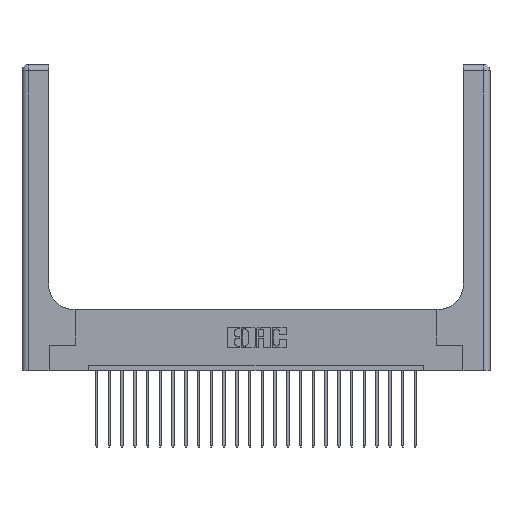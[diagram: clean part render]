
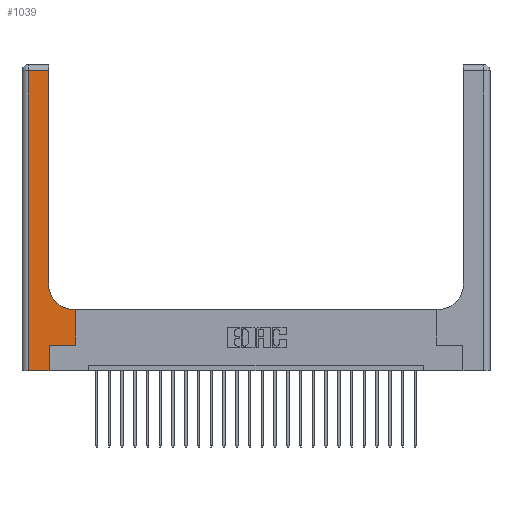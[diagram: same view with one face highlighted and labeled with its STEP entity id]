
A CAD part, top view. The second image highlights one B-rep face of the part: STEP entity #1039.
In plain terms, the highlighted planar face has unit normal (0, 0, 1).
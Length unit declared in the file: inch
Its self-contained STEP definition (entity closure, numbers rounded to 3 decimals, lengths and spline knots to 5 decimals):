
#389 = VERTEX_POINT ( 'NONE', #12969 ) ;
#565 = DIRECTION ( 'NONE',  ( 1., 0., 0. ) ) ;
#596 = EDGE_CURVE ( 'NONE', #2358, #16063, #3542, .T. ) ;
#1039 = ADVANCED_FACE ( 'NONE', ( #17517 ), #15504, .F. ) ;
#1702 = AXIS2_PLACEMENT_3D ( 'NONE', #22422, #6206, #7999 ) ;
#2172 = VECTOR ( 'NONE', #17030, 39.37008 ) ;
#2254 = EDGE_CURVE ( 'NONE', #389, #21819, #23244, .T. ) ;
#2358 = VERTEX_POINT ( 'NONE', #20498 ) ;
#2521 = DIRECTION ( 'NONE',  ( 0., 1., 0. ) ) ;
#2607 = CARTESIAN_POINT ( 'NONE',  ( 0., 0., 0.37 ) ) ;
#3182 = DIRECTION ( 'NONE',  ( 0., 1., 0. ) ) ;
#3448 = EDGE_CURVE ( 'NONE', #3880, #2358, #19218, .T. ) ;
#3542 = LINE ( 'NONE', #15411, #4671 ) ;
#3593 = ORIENTED_EDGE ( 'NONE', *, *, #3448, .T. ) ;
#3880 = VERTEX_POINT ( 'NONE', #18646 ) ;
#4174 = VERTEX_POINT ( 'NONE', #15863 ) ;
#4275 = CARTESIAN_POINT ( 'NONE',  ( 0.265, 0.25, 0.37 ) ) ;
#4594 = CARTESIAN_POINT ( 'NONE',  ( 0., 3., 0.37 ) ) ;
#4671 = VECTOR ( 'NONE', #2521, 39.37008 ) ;
#5484 = VECTOR ( 'NONE', #18751, 39.37008 ) ;
#5961 = VECTOR ( 'NONE', #6491, 39.37008 ) ;
#5964 = EDGE_CURVE ( 'NONE', #13296, #11748, #10240, .T. ) ;
#5990 = ORIENTED_EDGE ( 'NONE', *, *, #5964, .T. ) ;
#6074 = EDGE_CURVE ( 'NONE', #4174, #13296, #15674, .T. ) ;
#6206 = DIRECTION ( 'NONE',  ( 0., 0., -1. ) ) ;
#6491 = DIRECTION ( 'NONE',  ( 0., -1., 0. ) ) ;
#7997 = DIRECTION ( 'NONE',  ( -1., 0., 0. ) ) ;
#7999 = DIRECTION ( 'NONE',  ( 1., 0., 0. ) ) ;
#8484 = ORIENTED_EDGE ( 'NONE', *, *, #16014, .T. ) ;
#8502 = ORIENTED_EDGE ( 'NONE', *, *, #10331, .T. ) ;
#8885 = LINE ( 'NONE', #20473, #5484 ) ;
#8945 = LINE ( 'NONE', #4275, #13223 ) ;
#10072 = DIRECTION ( 'NONE',  ( -1., 0., 0. ) ) ;
#10240 = LINE ( 'NONE', #15080, #22770 ) ;
#10331 = EDGE_CURVE ( 'NONE', #11748, #18157, #20319, .T. ) ;
#11748 = VERTEX_POINT ( 'NONE', #16705 ) ;
#12388 = CARTESIAN_POINT ( 'NONE',  ( 0.26, 0.85, 0.37 ) ) ;
#12969 = CARTESIAN_POINT ( 'NONE',  ( 0.26, 2.94, 0.37 ) ) ;
#13201 = CARTESIAN_POINT ( 'NONE',  ( 0.528, 0.6, 0.37 ) ) ;
#13223 = VECTOR ( 'NONE', #565, 39.37008 ) ;
#13296 = VERTEX_POINT ( 'NONE', #13201 ) ;
#14224 = EDGE_CURVE ( 'NONE', #16063, #4174, #8945, .T. ) ;
#14757 = VECTOR ( 'NONE', #7997, 39.37008 ) ;
#14937 = ORIENTED_EDGE ( 'NONE', *, *, #596, .T. ) ;
#15080 = CARTESIAN_POINT ( 'NONE',  ( 0.26, 0.6, 0.37 ) ) ;
#15192 = CARTESIAN_POINT ( 'NONE',  ( 0., 2.94, 0.37 ) ) ;
#15411 = CARTESIAN_POINT ( 'NONE',  ( 0.265, 0., 0.37 ) ) ;
#15504 = PLANE ( 'NONE',  #15603 ) ;
#15603 = AXIS2_PLACEMENT_3D ( 'NONE', #4594, #17350, #10072 ) ;
#15674 = LINE ( 'NONE', #16080, #16852 ) ;
#15863 = CARTESIAN_POINT ( 'NONE',  ( 0.528, 0.25, 0.37 ) ) ;
#15875 = ORIENTED_EDGE ( 'NONE', *, *, #2254, .T. ) ;
#16014 = EDGE_CURVE ( 'NONE', #18157, #389, #8885, .T. ) ;
#16063 = VERTEX_POINT ( 'NONE', #19441 ) ;
#16080 = CARTESIAN_POINT ( 'NONE',  ( 0.528, 0.25, 0.37 ) ) ;
#16152 = ORIENTED_EDGE ( 'NONE', *, *, #17862, .T. ) ;
#16232 = LINE ( 'NONE', #17707, #5961 ) ;
#16694 = ORIENTED_EDGE ( 'NONE', *, *, #14224, .T. ) ;
#16705 = CARTESIAN_POINT ( 'NONE',  ( 0.51, 0.6, 0.37 ) ) ;
#16852 = VECTOR ( 'NONE', #3182, 39.37008 ) ;
#17030 = DIRECTION ( 'NONE',  ( 1., 0., 0. ) ) ;
#17350 = DIRECTION ( 'NONE',  ( 0., 0., -1. ) ) ;
#17517 = FACE_OUTER_BOUND ( 'NONE', #18189, .T. ) ;
#17707 = CARTESIAN_POINT ( 'NONE',  ( 0.06, 3., 0.37 ) ) ;
#17862 = EDGE_CURVE ( 'NONE', #21819, #3880, #16232, .T. ) ;
#18157 = VERTEX_POINT ( 'NONE', #12388 ) ;
#18189 = EDGE_LOOP ( 'NONE', ( #8484, #15875, #16152, #3593, #14937, #16694, #22482, #5990, #8502 ) ) ;
#18361 = CARTESIAN_POINT ( 'NONE',  ( 0.06, 2.94, 0.37 ) ) ;
#18646 = CARTESIAN_POINT ( 'NONE',  ( 0.06, 0., 0.37 ) ) ;
#18751 = DIRECTION ( 'NONE',  ( 0., 1., 0. ) ) ;
#18883 = DIRECTION ( 'NONE',  ( -1., 0., 0. ) ) ;
#19218 = LINE ( 'NONE', #2607, #2172 ) ;
#19441 = CARTESIAN_POINT ( 'NONE',  ( 0.265, 0.25, 0.37 ) ) ;
#20319 = CIRCLE ( 'NONE', #1702, 0.25 ) ;
#20473 = CARTESIAN_POINT ( 'NONE',  ( 0.26, 3., 0.37 ) ) ;
#20498 = CARTESIAN_POINT ( 'NONE',  ( 0.265, 0., 0.37 ) ) ;
#21819 = VERTEX_POINT ( 'NONE', #18361 ) ;
#22422 = CARTESIAN_POINT ( 'NONE',  ( 0.51, 0.85, 0.37 ) ) ;
#22482 = ORIENTED_EDGE ( 'NONE', *, *, #6074, .T. ) ;
#22770 = VECTOR ( 'NONE', #18883, 39.37008 ) ;
#23244 = LINE ( 'NONE', #15192, #14757 ) ;
